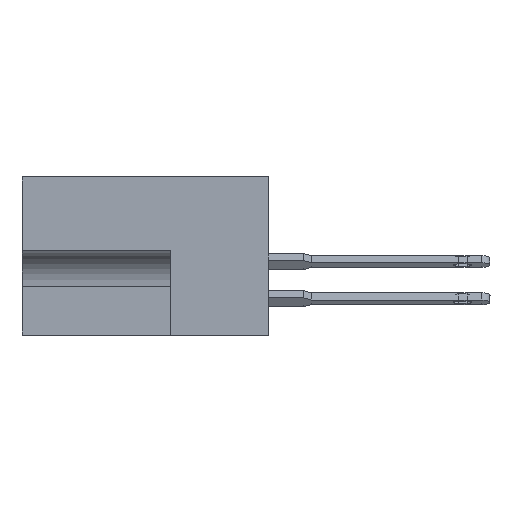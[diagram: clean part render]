
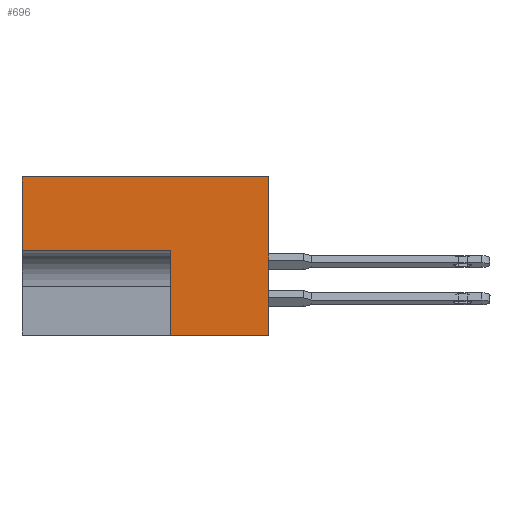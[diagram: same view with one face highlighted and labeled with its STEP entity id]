
A CAD part, left-side view. The second image highlights one B-rep face of the part: STEP entity #696.
In plain terms, the highlighted planar face has unit normal (-1, 0, 0).
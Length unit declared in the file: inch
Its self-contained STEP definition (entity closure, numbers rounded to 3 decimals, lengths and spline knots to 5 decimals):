
#696 = ADVANCED_FACE ( 'NONE', ( #2955 ), #8398, .F. ) ;
#855 = DIRECTION ( 'NONE',  ( 0., 0., 1. ) ) ;
#1196 = DIRECTION ( 'NONE',  ( 0., 0., 1. ) ) ;
#1592 = DIRECTION ( 'NONE',  ( 1., 0., 0. ) ) ;
#1682 = LINE ( 'NONE', #19078, #17923 ) ;
#1699 = VERTEX_POINT ( 'NONE', #6199 ) ;
#2000 = VERTEX_POINT ( 'NONE', #26311 ) ;
#2659 = CARTESIAN_POINT ( 'NONE',  ( 0., 0., -0.531 ) ) ;
#2955 = FACE_OUTER_BOUND ( 'NONE', #23075, .T. ) ;
#6178 = CARTESIAN_POINT ( 'NONE',  ( 0., 0.328, -0.531 ) ) ;
#6199 = CARTESIAN_POINT ( 'NONE',  ( 0., 0.828, 0. ) ) ;
#6270 = DIRECTION ( 'NONE',  ( 0., -1., 0. ) ) ;
#8054 = ORIENTED_EDGE ( 'NONE', *, *, #12115, .F. ) ;
#8081 = VERTEX_POINT ( 'NONE', #24475 ) ;
#8155 = VECTOR ( 'NONE', #855, 39.37008 ) ;
#8390 = ORIENTED_EDGE ( 'NONE', *, *, #17105, .F. ) ;
#8398 = PLANE ( 'NONE',  #18841 ) ;
#9798 = DIRECTION ( 'NONE',  ( 0., 1., 0. ) ) ;
#10183 = VECTOR ( 'NONE', #21171, 39.37008 ) ;
#10758 = EDGE_CURVE ( 'NONE', #11872, #15449, #15358, .T. ) ;
#10802 = LINE ( 'NONE', #10949, #25258 ) ;
#10949 = CARTESIAN_POINT ( 'NONE',  ( 0., 0.453, 0. ) ) ;
#11872 = VERTEX_POINT ( 'NONE', #6178 ) ;
#12115 = EDGE_CURVE ( 'NONE', #2000, #13205, #18245, .T. ) ;
#13205 = VERTEX_POINT ( 'NONE', #29729 ) ;
#13322 = LINE ( 'NONE', #17693, #8155 ) ;
#15358 = LINE ( 'NONE', #18684, #10183 ) ;
#15449 = VERTEX_POINT ( 'NONE', #2659 ) ;
#15704 = ORIENTED_EDGE ( 'NONE', *, *, #10758, .T. ) ;
#17105 = EDGE_CURVE ( 'NONE', #13205, #1699, #1682, .T. ) ;
#17149 = ORIENTED_EDGE ( 'NONE', *, *, #18966, .T. ) ;
#17693 = CARTESIAN_POINT ( 'NONE',  ( 0., 0.328, -0.531 ) ) ;
#17914 = ORIENTED_EDGE ( 'NONE', *, *, #19627, .F. ) ;
#17923 = VECTOR ( 'NONE', #21659, 39.37008 ) ;
#18245 = LINE ( 'NONE', #25864, #19733 ) ;
#18684 = CARTESIAN_POINT ( 'NONE',  ( 0., 0.453, -0.531 ) ) ;
#18841 = AXIS2_PLACEMENT_3D ( 'NONE', #25199, #1592, #29931 ) ;
#18966 = EDGE_CURVE ( 'NONE', #15449, #8081, #30048, .T. ) ;
#19078 = CARTESIAN_POINT ( 'NONE',  ( 0., 0.828, 0. ) ) ;
#19627 = EDGE_CURVE ( 'NONE', #11872, #2000, #13322, .T. ) ;
#19733 = VECTOR ( 'NONE', #9798, 39.37008 ) ;
#21171 = DIRECTION ( 'NONE',  ( 0., -1., 0. ) ) ;
#21500 = VECTOR ( 'NONE', #1196, 39.37008 ) ;
#21659 = DIRECTION ( 'NONE',  ( 0., 0., 1. ) ) ;
#22856 = ORIENTED_EDGE ( 'NONE', *, *, #29700, .F. ) ;
#23075 = EDGE_LOOP ( 'NONE', ( #8390, #8054, #17914, #15704, #17149, #22856 ) ) ;
#24475 = CARTESIAN_POINT ( 'NONE',  ( 0., 0., 0. ) ) ;
#25199 = CARTESIAN_POINT ( 'NONE',  ( 0., 0.453, 0. ) ) ;
#25210 = CARTESIAN_POINT ( 'NONE',  ( 0., 0., 0. ) ) ;
#25258 = VECTOR ( 'NONE', #6270, 39.37008 ) ;
#25864 = CARTESIAN_POINT ( 'NONE',  ( 0., 0.328, -0.248 ) ) ;
#26311 = CARTESIAN_POINT ( 'NONE',  ( 0., 0.328, -0.248 ) ) ;
#29700 = EDGE_CURVE ( 'NONE', #1699, #8081, #10802, .T. ) ;
#29729 = CARTESIAN_POINT ( 'NONE',  ( 0., 0.828, -0.248 ) ) ;
#29931 = DIRECTION ( 'NONE',  ( 0., 0., -1. ) ) ;
#30048 = LINE ( 'NONE', #25210, #21500 ) ;
